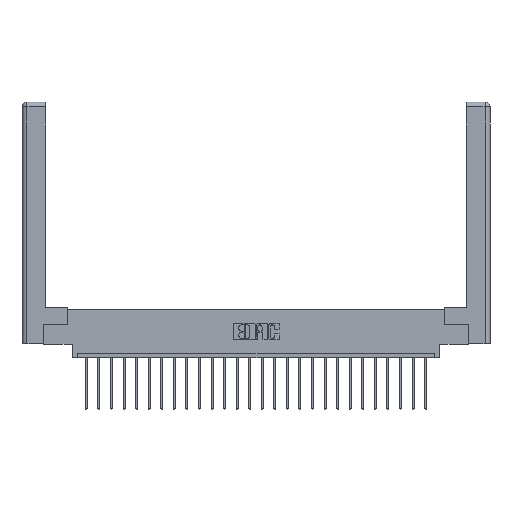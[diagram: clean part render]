
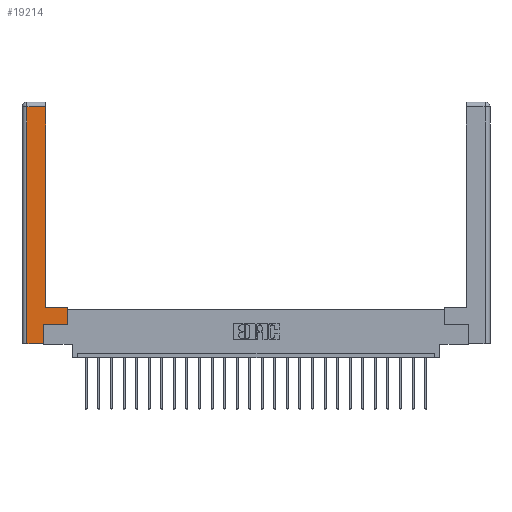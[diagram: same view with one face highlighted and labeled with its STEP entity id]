
A CAD part, top view. The second image highlights one B-rep face of the part: STEP entity #19214.
In plain terms, the highlighted planar face has unit normal (0, 0, 1).
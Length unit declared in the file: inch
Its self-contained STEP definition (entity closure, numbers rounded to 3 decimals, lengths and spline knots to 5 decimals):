
#368 = CARTESIAN_POINT ( 'NONE',  ( 0.295, 0.45, 0. ) ) ;
#622 = CARTESIAN_POINT ( 'NONE',  ( 0., 0., 0. ) ) ;
#789 = LINE ( 'NONE', #13204, #15810 ) ;
#895 = DIRECTION ( 'NONE',  ( 0., 1., 0. ) ) ;
#1437 = CARTESIAN_POINT ( 'NONE',  ( 0.295, 0.45, 0. ) ) ;
#1879 = DIRECTION ( 'NONE',  ( 0., 1., 0. ) ) ;
#2092 = CARTESIAN_POINT ( 'NONE',  ( 0.565, 0.245, 0. ) ) ;
#2221 = CARTESIAN_POINT ( 'NONE',  ( 0.565, 0.245, 0. ) ) ;
#2759 = LINE ( 'NONE', #6658, #12887 ) ;
#3038 = DIRECTION ( 'NONE',  ( -1., 0., 0. ) ) ;
#3441 = ORIENTED_EDGE ( 'NONE', *, *, #21749, .T. ) ;
#3596 = VECTOR ( 'NONE', #13292, 39.37008 ) ;
#3599 = DIRECTION ( 'NONE',  ( -1., 0., 0. ) ) ;
#3792 = CARTESIAN_POINT ( 'NONE',  ( 0.265, 0., 0. ) ) ;
#3857 = EDGE_CURVE ( 'NONE', #15230, #14928, #17365, .T. ) ;
#3971 = EDGE_CURVE ( 'NONE', #19238, #13042, #19222, .T. ) ;
#4250 = DIRECTION ( 'NONE',  ( 1., 0., 0. ) ) ;
#4828 = EDGE_LOOP ( 'NONE', ( #23049, #6335, #9644, #3441, #9302, #11971, #20555, #22124 ) ) ;
#5049 = CARTESIAN_POINT ( 'NONE',  ( 0.295, 2.94, 0. ) ) ;
#5409 = DIRECTION ( 'NONE',  ( 0., -1., 0. ) ) ;
#5698 = CARTESIAN_POINT ( 'NONE',  ( 0.0615, 0., 0. ) ) ;
#5971 = DIRECTION ( 'NONE',  ( 1., 0., 0. ) ) ;
#6250 = CARTESIAN_POINT ( 'NONE',  ( 0.0615, 2.94, 0. ) ) ;
#6335 = ORIENTED_EDGE ( 'NONE', *, *, #11783, .T. ) ;
#6658 = CARTESIAN_POINT ( 'NONE',  ( 0.295, 3., 0. ) ) ;
#7120 = FACE_OUTER_BOUND ( 'NONE', #4828, .T. ) ;
#7886 = LINE ( 'NONE', #14312, #17680 ) ;
#8220 = CARTESIAN_POINT ( 'NONE',  ( 0.265, 0.245, 0. ) ) ;
#8709 = PLANE ( 'NONE',  #12652 ) ;
#8790 = VERTEX_POINT ( 'NONE', #2221 ) ;
#9232 = CARTESIAN_POINT ( 'NONE',  ( 0.565, 0.45, 0. ) ) ;
#9302 = ORIENTED_EDGE ( 'NONE', *, *, #3857, .T. ) ;
#9607 = CARTESIAN_POINT ( 'NONE',  ( 0.0615, 2.94, 0. ) ) ;
#9644 = ORIENTED_EDGE ( 'NONE', *, *, #17164, .T. ) ;
#10695 = DIRECTION ( 'NONE',  ( 0., 0., -1. ) ) ;
#11004 = LINE ( 'NONE', #13649, #24460 ) ;
#11783 = EDGE_CURVE ( 'NONE', #17028, #14558, #18355, .T. ) ;
#11971 = ORIENTED_EDGE ( 'NONE', *, *, #12357, .T. ) ;
#12357 = EDGE_CURVE ( 'NONE', #14928, #8790, #21391, .T. ) ;
#12525 = VECTOR ( 'NONE', #5971, 39.37008 ) ;
#12652 = AXIS2_PLACEMENT_3D ( 'NONE', #622, #10695, #3038 ) ;
#12887 = VECTOR ( 'NONE', #895, 39.37008 ) ;
#13042 = VERTEX_POINT ( 'NONE', #368 ) ;
#13204 = CARTESIAN_POINT ( 'NONE',  ( 0.0615, 0., 0. ) ) ;
#13292 = DIRECTION ( 'NONE',  ( -1., 0., 0. ) ) ;
#13649 = CARTESIAN_POINT ( 'NONE',  ( 0.565, 0.45, 0. ) ) ;
#14312 = CARTESIAN_POINT ( 'NONE',  ( 0.265, 0., 0. ) ) ;
#14558 = VERTEX_POINT ( 'NONE', #6250 ) ;
#14928 = VERTEX_POINT ( 'NONE', #20662 ) ;
#15230 = VERTEX_POINT ( 'NONE', #3792 ) ;
#15810 = VECTOR ( 'NONE', #5409, 39.37008 ) ;
#15899 = VECTOR ( 'NONE', #3599, 39.37008 ) ;
#17028 = VERTEX_POINT ( 'NONE', #5049 ) ;
#17164 = EDGE_CURVE ( 'NONE', #14558, #20417, #789, .T. ) ;
#17365 = LINE ( 'NONE', #8220, #21960 ) ;
#17569 = EDGE_CURVE ( 'NONE', #13042, #17028, #2759, .T. ) ;
#17680 = VECTOR ( 'NONE', #4250, 39.37008 ) ;
#18355 = LINE ( 'NONE', #9607, #15899 ) ;
#19214 = ADVANCED_FACE ( 'NONE', ( #7120 ), #8709, .F. ) ;
#19222 = LINE ( 'NONE', #1437, #3596 ) ;
#19238 = VERTEX_POINT ( 'NONE', #9232 ) ;
#20417 = VERTEX_POINT ( 'NONE', #5698 ) ;
#20555 = ORIENTED_EDGE ( 'NONE', *, *, #24225, .T. ) ;
#20662 = CARTESIAN_POINT ( 'NONE',  ( 0.265, 0.245, 0. ) ) ;
#21391 = LINE ( 'NONE', #2092, #12525 ) ;
#21749 = EDGE_CURVE ( 'NONE', #20417, #15230, #7886, .T. ) ;
#21960 = VECTOR ( 'NONE', #23881, 39.37008 ) ;
#22124 = ORIENTED_EDGE ( 'NONE', *, *, #3971, .T. ) ;
#23049 = ORIENTED_EDGE ( 'NONE', *, *, #17569, .T. ) ;
#23881 = DIRECTION ( 'NONE',  ( 0., 1., 0. ) ) ;
#24225 = EDGE_CURVE ( 'NONE', #8790, #19238, #11004, .T. ) ;
#24460 = VECTOR ( 'NONE', #1879, 39.37008 ) ;
